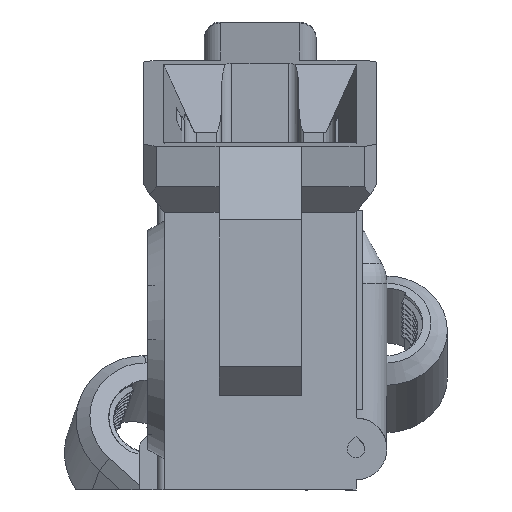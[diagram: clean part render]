
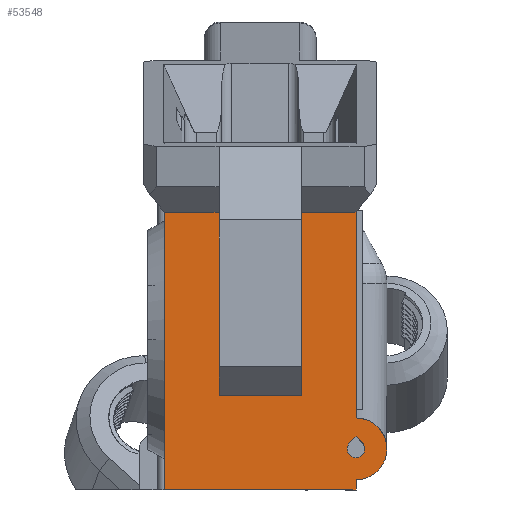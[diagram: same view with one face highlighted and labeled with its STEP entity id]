
A CAD part, left-side view. The second image highlights one B-rep face of the part: STEP entity #53548.
In plain terms, the highlighted planar face has unit normal (-1, 0, 0).
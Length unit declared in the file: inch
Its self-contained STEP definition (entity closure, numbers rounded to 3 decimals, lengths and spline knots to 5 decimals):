
#218 = FACE_OUTER_BOUND ( 'NONE', #32263, .T. ) ;
#1110 = DIRECTION ( 'NONE',  ( 0., 0., -1. ) ) ;
#3968 = CARTESIAN_POINT ( 'NONE',  ( -3.562, 1.4856, 1.82821 ) ) ;
#4480 = CARTESIAN_POINT ( 'NONE',  ( -3.562, 0.3196, 1.15376 ) ) ;
#5786 = DIRECTION ( 'NONE',  ( 0., 0., -1. ) ) ;
#6149 = ORIENTED_EDGE ( 'NONE', *, *, #69328, .F. ) ;
#10431 = LINE ( 'NONE', #173127, #178074 ) ;
#11765 = CARTESIAN_POINT ( 'NONE',  ( -3.562, 0.3196, 1.07821 ) ) ;
#13377 = VERTEX_POINT ( 'NONE', #47956 ) ;
#13721 = LINE ( 'NONE', #91689, #68240 ) ;
#16199 = EDGE_CURVE ( 'NONE', #93914, #109650, #10431, .T. ) ;
#22691 = EDGE_CURVE ( 'NONE', #71616, #171185, #145077, .T. ) ;
#23173 = ORIENTED_EDGE ( 'NONE', *, *, #169651, .T. ) ;
#26105 = EDGE_CURVE ( 'NONE', #52777, #171185, #13721, .T. ) ;
#26782 = CARTESIAN_POINT ( 'NONE',  ( -3.562, 0.35737, 1.11598 ) ) ;
#28317 = CARTESIAN_POINT ( 'NONE',  ( -3.562, 1.1526, 1.40321 ) ) ;
#28984 = VECTOR ( 'NONE', #128494, 39.37008 ) ;
#31591 = ORIENTED_EDGE ( 'NONE', *, *, #95082, .T. ) ;
#32263 = EDGE_LOOP ( 'NONE', ( #23173, #31591, #125949, #119662, #101190, #97158, #96345, #64500, #6149, #169273 ) ) ;
#39467 = CARTESIAN_POINT ( 'NONE',  ( -3.562, 0.6526, 2.51798 ) ) ;
#41029 = CARTESIAN_POINT ( 'NONE',  ( -3.562, 0.3196, 1.82821 ) ) ;
#43611 = EDGE_CURVE ( 'NONE', #117385, #60048, #67243, .T. ) ;
#46590 = DIRECTION ( 'NONE',  ( 0., 0., 1. ) ) ;
#47956 = CARTESIAN_POINT ( 'NONE',  ( -3.562, 0.28182, 1.11598 ) ) ;
#48667 = DIRECTION ( 'NONE',  ( 0., 0.707, 0.707 ) ) ;
#49150 = AXIS2_PLACEMENT_3D ( 'NONE', #85758, #122893, #1110 ) ;
#49563 = DIRECTION ( 'NONE',  ( 0., 0.707, -0.707 ) ) ;
#50225 = DIRECTION ( 'NONE',  ( 0., -1., 0. ) ) ;
#52777 = VERTEX_POINT ( 'NONE', #28317 ) ;
#53548 = ADVANCED_FACE ( 'NONE', ( #218, #159205 ), #156715, .F. ) ;
#53657 = VECTOR ( 'NONE', #48667, 39.37008 ) ;
#58997 = AXIS2_PLACEMENT_3D ( 'NONE', #169554, #86213, #46590 ) ;
#60048 = VERTEX_POINT ( 'NONE', #110311 ) ;
#63177 = ORIENTED_EDGE ( 'NONE', *, *, #83668, .F. ) ;
#63310 = LINE ( 'NONE', #3968, #96004 ) ;
#64500 = ORIENTED_EDGE ( 'NONE', *, *, #26105, .F. ) ;
#65444 = EDGE_CURVE ( 'NONE', #117385, #165442, #170294, .T. ) ;
#65905 = CARTESIAN_POINT ( 'NONE',  ( -3.562, 1.1526, 0.82821 ) ) ;
#67243 = LINE ( 'NONE', #41029, #178289 ) ;
#67771 = DIRECTION ( 'NONE',  ( -1., 0., 0. ) ) ;
#68240 = VECTOR ( 'NONE', #50225, 39.37008 ) ;
#68824 = ORIENTED_EDGE ( 'NONE', *, *, #122806, .F. ) ;
#69328 = EDGE_CURVE ( 'NONE', #166568, #52777, #153660, .T. ) ;
#71572 = AXIS2_PLACEMENT_3D ( 'NONE', #11765, #67771, #109182 ) ;
#71616 = VERTEX_POINT ( 'NONE', #39467 ) ;
#72240 = VERTEX_POINT ( 'NONE', #124590 ) ;
#72935 = CARTESIAN_POINT ( 'NONE',  ( -3.562, 0.6526, 2.51798 ) ) ;
#74826 = DIRECTION ( 'NONE',  ( 0., 0., -1. ) ) ;
#75491 = CARTESIAN_POINT ( 'NONE',  ( -3.562, 0.28182, 1.11598 ) ) ;
#78137 = CARTESIAN_POINT ( 'NONE',  ( -3.562, 0.3196, 1.26621 ) ) ;
#83668 = EDGE_CURVE ( 'NONE', #109650, #165091, #151553, .T. ) ;
#85758 = CARTESIAN_POINT ( 'NONE',  ( -3.562, 0.3196, 1.07821 ) ) ;
#86213 = DIRECTION ( 'NONE',  ( 1., 0., 0. ) ) ;
#88337 = EDGE_CURVE ( 'NONE', #166568, #72240, #170486, .T. ) ;
#89363 = LINE ( 'NONE', #102860, #163294 ) ;
#90197 = CARTESIAN_POINT ( 'NONE',  ( -3.562, 0.6526, 1.40321 ) ) ;
#90371 = DIRECTION ( 'NONE',  ( 0., -1., 0. ) ) ;
#91133 = EDGE_CURVE ( 'NONE', #133927, #71616, #89363, .T. ) ;
#91689 = CARTESIAN_POINT ( 'NONE',  ( -3.562, 2.4558, 1.40321 ) ) ;
#92987 = LINE ( 'NONE', #75491, #53657 ) ;
#93914 = VERTEX_POINT ( 'NONE', #4480 ) ;
#95082 = EDGE_CURVE ( 'NONE', #151314, #60048, #177790, .T. ) ;
#96004 = VECTOR ( 'NONE', #5786, 39.37008 ) ;
#96345 = ORIENTED_EDGE ( 'NONE', *, *, #22691, .T. ) ;
#97158 = ORIENTED_EDGE ( 'NONE', *, *, #91133, .T. ) ;
#97366 = VECTOR ( 'NONE', #90371, 39.37008 ) ;
#100635 = EDGE_CURVE ( 'NONE', #133927, #165442, #170158, .T. ) ;
#101190 = ORIENTED_EDGE ( 'NONE', *, *, #100635, .F. ) ;
#101533 = VECTOR ( 'NONE', #163870, 39.37008 ) ;
#101704 = AXIS2_PLACEMENT_3D ( 'NONE', #129002, #173331, #74826 ) ;
#102344 = CARTESIAN_POINT ( 'NONE',  ( -3.562, -0.1474, 2.51798 ) ) ;
#102860 = CARTESIAN_POINT ( 'NONE',  ( -3.562, -0.1474, 2.51798 ) ) ;
#106721 = CARTESIAN_POINT ( 'NONE',  ( -3.562, 0.3196, 3.25138 ) ) ;
#107957 = EDGE_LOOP ( 'NONE', ( #63177, #108625, #145843, #68824 ) ) ;
#108625 = ORIENTED_EDGE ( 'NONE', *, *, #16199, .F. ) ;
#109182 = DIRECTION ( 'NONE',  ( 0., 0., 1. ) ) ;
#109650 = VERTEX_POINT ( 'NONE', #26782 ) ;
#110311 = CARTESIAN_POINT ( 'NONE',  ( -3.562, 0.3196, 0.82821 ) ) ;
#115709 = VECTOR ( 'NONE', #178427, 39.37008 ) ;
#117385 = VERTEX_POINT ( 'NONE', #156906 ) ;
#119662 = ORIENTED_EDGE ( 'NONE', *, *, #65444, .T. ) ;
#121162 = VECTOR ( 'NONE', #144137, 39.37008 ) ;
#122806 = EDGE_CURVE ( 'NONE', #165091, #13377, #155089, .T. ) ;
#122893 = DIRECTION ( 'NONE',  ( -1., 0., 0. ) ) ;
#124590 = CARTESIAN_POINT ( 'NONE',  ( -3.562, 1.4856, 2.51798 ) ) ;
#125949 = ORIENTED_EDGE ( 'NONE', *, *, #43611, .F. ) ;
#128494 = DIRECTION ( 'NONE',  ( 0., 1., 0. ) ) ;
#129002 = CARTESIAN_POINT ( 'NONE',  ( -3.562, 0.3196, 1.07821 ) ) ;
#133927 = VERTEX_POINT ( 'NONE', #160842 ) ;
#140359 = CARTESIAN_POINT ( 'NONE',  ( -3.562, 1.4856, 0.82821 ) ) ;
#140724 = CARTESIAN_POINT ( 'NONE',  ( -3.562, 1.1526, 2.51798 ) ) ;
#143570 = DIRECTION ( 'NONE',  ( 0., 1., 0. ) ) ;
#144137 = DIRECTION ( 'NONE',  ( 0., 0., -1. ) ) ;
#145077 = LINE ( 'NONE', #72935, #121162 ) ;
#145687 = CARTESIAN_POINT ( 'NONE',  ( -3.562, 0.6526, 0.82821 ) ) ;
#145843 = ORIENTED_EDGE ( 'NONE', *, *, #158107, .F. ) ;
#151314 = VERTEX_POINT ( 'NONE', #140359 ) ;
#151553 = CIRCLE ( 'NONE', #101704, 0.05342 ) ;
#153660 = LINE ( 'NONE', #65905, #101533 ) ;
#155089 = CIRCLE ( 'NONE', #49150, 0.05342 ) ;
#156715 = PLANE ( 'NONE',  #58997 ) ;
#156906 = CARTESIAN_POINT ( 'NONE',  ( -3.562, 0.3196, 0.89021 ) ) ;
#158107 = EDGE_CURVE ( 'NONE', #13377, #93914, #92987, .T. ) ;
#159205 = FACE_BOUND ( 'NONE', #107957, .T. ) ;
#160842 = CARTESIAN_POINT ( 'NONE',  ( -3.562, 0.3196, 2.51798 ) ) ;
#162175 = CARTESIAN_POINT ( 'NONE',  ( -3.562, 0.3196, 1.02479 ) ) ;
#163294 = VECTOR ( 'NONE', #143570, 39.37008 ) ;
#163870 = DIRECTION ( 'NONE',  ( 0., 0., -1. ) ) ;
#165091 = VERTEX_POINT ( 'NONE', #162175 ) ;
#165442 = VERTEX_POINT ( 'NONE', #78137 ) ;
#166568 = VERTEX_POINT ( 'NONE', #140724 ) ;
#166998 = DIRECTION ( 'NONE',  ( 0., 0., -1. ) ) ;
#169273 = ORIENTED_EDGE ( 'NONE', *, *, #88337, .T. ) ;
#169554 = CARTESIAN_POINT ( 'NONE',  ( -3.562, 0.6526, 1.82821 ) ) ;
#169651 = EDGE_CURVE ( 'NONE', #72240, #151314, #63310, .T. ) ;
#170158 = LINE ( 'NONE', #106721, #115709 ) ;
#170294 = CIRCLE ( 'NONE', #71572, 0.188 ) ;
#170486 = LINE ( 'NONE', #102344, #28984 ) ;
#171185 = VERTEX_POINT ( 'NONE', #90197 ) ;
#173127 = CARTESIAN_POINT ( 'NONE',  ( -3.562, 0.3196, 1.15376 ) ) ;
#173331 = DIRECTION ( 'NONE',  ( -1., 0., 0. ) ) ;
#177790 = LINE ( 'NONE', #145687, #97366 ) ;
#178074 = VECTOR ( 'NONE', #49563, 39.37008 ) ;
#178289 = VECTOR ( 'NONE', #166998, 39.37008 ) ;
#178427 = DIRECTION ( 'NONE',  ( 0., 0., -1. ) ) ;
